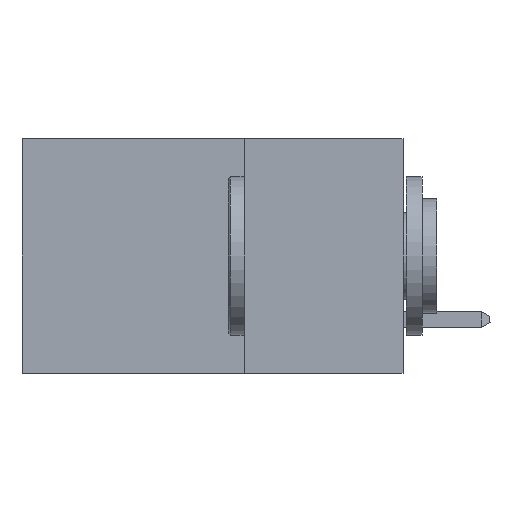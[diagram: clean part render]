
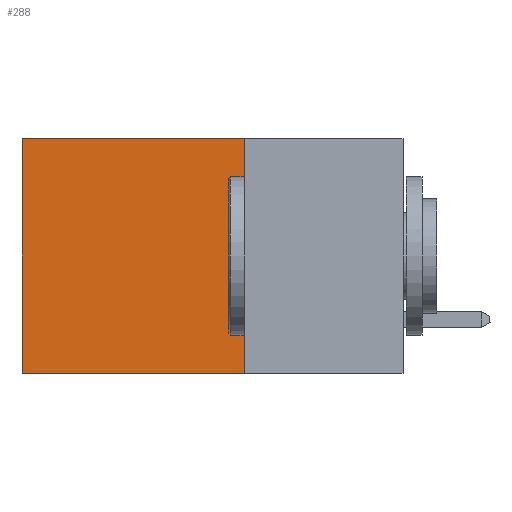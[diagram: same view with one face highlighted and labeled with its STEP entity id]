
A CAD part, left-side view. The second image highlights one B-rep face of the part: STEP entity #288.
In plain terms, the highlighted planar face has unit normal (-1, 0, 0).
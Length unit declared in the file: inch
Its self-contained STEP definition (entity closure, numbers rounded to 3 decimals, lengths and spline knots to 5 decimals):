
#24 = EDGE_CURVE ( 'NONE', #8134, #4317, #12671, .T. ) ;
#288 = ADVANCED_FACE ( 'NONE', ( #17737 ), #5049, .F. ) ;
#542 = CARTESIAN_POINT ( 'NONE',  ( 0.2875, 0.25, 0. ) ) ;
#1114 = ORIENTED_EDGE ( 'NONE', *, *, #6548, .T. ) ;
#1592 = CARTESIAN_POINT ( 'NONE',  ( 0.2875, 0.25, 0. ) ) ;
#3589 = VECTOR ( 'NONE', #8375, 39.37008 ) ;
#3928 = CARTESIAN_POINT ( 'NONE',  ( 0.2875, 0.6, 0. ) ) ;
#4317 = VERTEX_POINT ( 'NONE', #27798 ) ;
#5049 = PLANE ( 'NONE',  #18373 ) ;
#5430 = CARTESIAN_POINT ( 'NONE',  ( 0.2875, 0.25, 0. ) ) ;
#5740 = CARTESIAN_POINT ( 'NONE',  ( 0.2875, 0.25, 0. ) ) ;
#6029 = VECTOR ( 'NONE', #19038, 39.37008 ) ;
#6548 = EDGE_CURVE ( 'NONE', #8134, #9123, #17451, .T. ) ;
#6906 = VECTOR ( 'NONE', #18893, 39.37008 ) ;
#8134 = VERTEX_POINT ( 'NONE', #5740 ) ;
#8375 = DIRECTION ( 'NONE',  ( 0., 1., 0. ) ) ;
#8886 = CARTESIAN_POINT ( 'NONE',  ( 0.2875, 0.25, -0.37 ) ) ;
#9123 = VERTEX_POINT ( 'NONE', #17495 ) ;
#10639 = ORIENTED_EDGE ( 'NONE', *, *, #11656, .F. ) ;
#11656 = EDGE_CURVE ( 'NONE', #4317, #18218, #13959, .T. ) ;
#12671 = LINE ( 'NONE', #1592, #6906 ) ;
#13959 = LINE ( 'NONE', #8886, #21751 ) ;
#15432 = DIRECTION ( 'NONE',  ( 0., 1., 0. ) ) ;
#15569 = DIRECTION ( 'NONE',  ( 1., 0., 0. ) ) ;
#17451 = LINE ( 'NONE', #5430, #3589 ) ;
#17495 = CARTESIAN_POINT ( 'NONE',  ( 0.2875, 0.6, 0. ) ) ;
#17737 = FACE_OUTER_BOUND ( 'NONE', #26507, .T. ) ;
#18218 = VERTEX_POINT ( 'NONE', #22313 ) ;
#18373 = AXIS2_PLACEMENT_3D ( 'NONE', #542, #15569, #20186 ) ;
#18893 = DIRECTION ( 'NONE',  ( 0., 0., -1. ) ) ;
#19038 = DIRECTION ( 'NONE',  ( 0., 0., -1. ) ) ;
#19265 = ORIENTED_EDGE ( 'NONE', *, *, #24, .F. ) ;
#20186 = DIRECTION ( 'NONE',  ( 0., 0., -1. ) ) ;
#21751 = VECTOR ( 'NONE', #15432, 39.37008 ) ;
#22313 = CARTESIAN_POINT ( 'NONE',  ( 0.2875, 0.6, -0.37 ) ) ;
#24767 = EDGE_CURVE ( 'NONE', #9123, #18218, #25616, .T. ) ;
#25616 = LINE ( 'NONE', #3928, #6029 ) ;
#26507 = EDGE_LOOP ( 'NONE', ( #27393, #10639, #19265, #1114 ) ) ;
#27393 = ORIENTED_EDGE ( 'NONE', *, *, #24767, .T. ) ;
#27798 = CARTESIAN_POINT ( 'NONE',  ( 0.2875, 0.25, -0.37 ) ) ;
